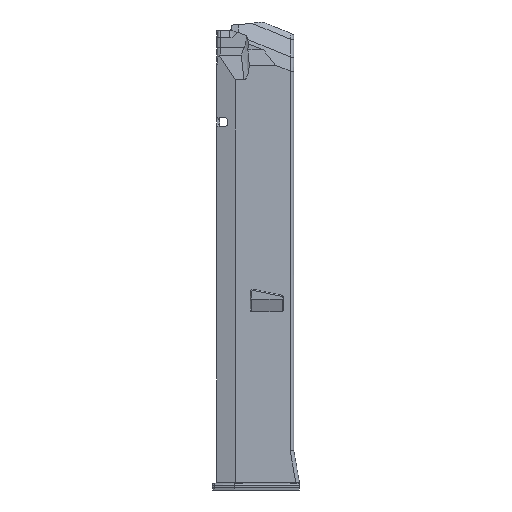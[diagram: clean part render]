
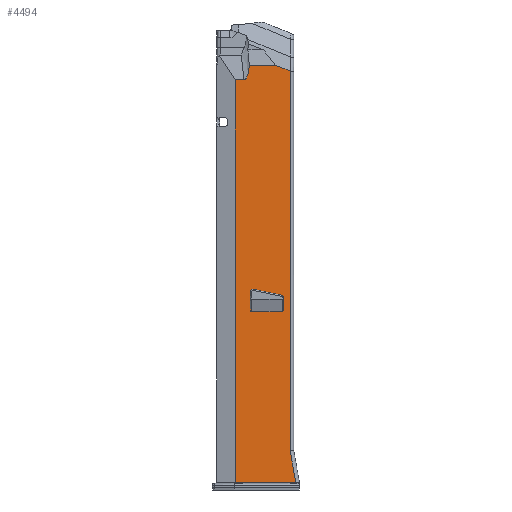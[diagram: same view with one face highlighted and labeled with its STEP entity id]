
A CAD part, left-side view. The second image highlights one B-rep face of the part: STEP entity #4494.
In plain terms, the highlighted planar face has unit normal (-1, 0, 0).
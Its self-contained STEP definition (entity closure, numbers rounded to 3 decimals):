
#103=FACE_BOUND('',#871,.T.);
#232=ELLIPSE('',#4677,1.005,1.);
#234=ELLIPSE('',#4680,1.005,1.);
#236=ELLIPSE('',#4683,1.463,0.503);
#240=ELLIPSE('',#4691,1.463,0.503);
#604=FACE_OUTER_BOUND('',#870,.T.);
#870=EDGE_LOOP('',(#4104,#4105,#4106,#4107,#4108,#4109,#4110,#4111));
#871=EDGE_LOOP('',(#4112,#4113,#4114,#4115,#4116,#4117,#4118,#4119));
#875=LINE('',#5754,#1214);
#882=LINE('',#5841,#1221);
#983=LINE('',#6915,#1322);
#989=LINE('',#6984,#1328);
#994=LINE('',#7002,#1333);
#1074=LINE('',#8695,#1413);
#1077=LINE('',#8703,#1416);
#1082=LINE('',#8725,#1421);
#1085=LINE('',#8741,#1424);
#1175=LINE('',#11174,#1514);
#1211=LINE('',#11465,#1550);
#1214=VECTOR('',#4813,10.);
#1221=VECTOR('',#4826,10.043);
#1322=VECTOR('',#5065,10.05);
#1328=VECTOR('',#5085,10.002);
#1333=VECTOR('',#5098,10.);
#1413=VECTOR('',#5338,10.05);
#1416=VECTOR('',#5343,10.);
#1421=VECTOR('',#5354,10.048);
#1424=VECTOR('',#5363,10.);
#1514=VECTOR('',#5635,10.05);
#1550=VECTOR('',#5731,10.);
#1559=B_SPLINE_CURVE_WITH_KNOTS('',3,(#5826,#5827,#5828,#5829,#5830,#5831,
#5832,#5833,#5834,#5835,#5836,#5837,#5838),.UNSPECIFIED.,.F.,.F.,(4,3,3,
3,4),(0.44,0.612,0.907,1.091,
1.202),.UNSPECIFIED.);
#1712=VERTEX_POINT('',#5748);
#1713=VERTEX_POINT('',#5753);
#1723=VERTEX_POINT('',#5821);
#1724=VERTEX_POINT('',#5840);
#1826=VERTEX_POINT('',#6840);
#1836=VERTEX_POINT('',#6914);
#1842=VERTEX_POINT('',#6982);
#1845=VERTEX_POINT('',#7001);
#1972=VERTEX_POINT('',#8691);
#1973=VERTEX_POINT('',#8693);
#1976=VERTEX_POINT('',#8700);
#1977=VERTEX_POINT('',#8702);
#1979=VERTEX_POINT('',#8717);
#1981=VERTEX_POINT('',#8723);
#1983=VERTEX_POINT('',#8734);
#1985=VERTEX_POINT('',#8739);
#2133=EDGE_CURVE('',#1713,#1712,#875,.T.);
#2146=EDGE_CURVE('',#1723,#1712,#1559,.F.);
#2147=EDGE_CURVE('',#1713,#1724,#882,.T.);
#2311=EDGE_CURVE('',#1826,#1836,#983,.T.);
#2324=EDGE_CURVE('',#1842,#1826,#989,.T.);
#2330=EDGE_CURVE('',#1845,#1836,#994,.T.);
#2510=EDGE_CURVE('',#1973,#1972,#1074,.T.);
#2513=EDGE_CURVE('',#1976,#1977,#1077,.T.);
#2517=EDGE_CURVE('',#1976,#1979,#232,.F.);
#2520=EDGE_CURVE('',#1981,#1979,#1082,.T.);
#2523=EDGE_CURVE('',#1981,#1983,#234,.F.);
#2525=EDGE_CURVE('',#1985,#1983,#1085,.T.);
#2528=EDGE_CURVE('',#1973,#1977,#236,.F.);
#2534=EDGE_CURVE('',#1985,#1972,#240,.F.);
#2744=EDGE_CURVE('',#1845,#1723,#1175,.T.);
#2799=EDGE_CURVE('',#1724,#1842,#1211,.T.);
#4104=ORIENTED_EDGE('',*,*,#2133,.T.);
#4105=ORIENTED_EDGE('',*,*,#2146,.F.);
#4106=ORIENTED_EDGE('',*,*,#2744,.F.);
#4107=ORIENTED_EDGE('',*,*,#2330,.T.);
#4108=ORIENTED_EDGE('',*,*,#2311,.F.);
#4109=ORIENTED_EDGE('',*,*,#2324,.F.);
#4110=ORIENTED_EDGE('',*,*,#2799,.F.);
#4111=ORIENTED_EDGE('',*,*,#2147,.F.);
#4112=ORIENTED_EDGE('',*,*,#2510,.F.);
#4113=ORIENTED_EDGE('',*,*,#2528,.T.);
#4114=ORIENTED_EDGE('',*,*,#2513,.F.);
#4115=ORIENTED_EDGE('',*,*,#2517,.T.);
#4116=ORIENTED_EDGE('',*,*,#2520,.F.);
#4117=ORIENTED_EDGE('',*,*,#2523,.T.);
#4118=ORIENTED_EDGE('',*,*,#2525,.F.);
#4119=ORIENTED_EDGE('',*,*,#2534,.T.);
#4242=PLANE('',#4803);
#4494=ADVANCED_FACE('',(#604,#103),#4242,.T.);
#4677=AXIS2_PLACEMENT_3D('',#8719,#5348,#5349);
#4680=AXIS2_PLACEMENT_3D('',#8736,#5358,#5359);
#4683=AXIS2_PLACEMENT_3D('',#8750,#5367,#5368);
#4691=AXIS2_PLACEMENT_3D('',#8932,#5383,#5384);
#4803=AXIS2_PLACEMENT_3D('',#11466,#5732,#5733);
#4813=DIRECTION('',(0.,1.,0.));
#4826=DIRECTION('',(0.,-0.925,-0.381));
#5065=DIRECTION('',(0.,1.,0.));
#5085=DIRECTION('',(0.,-0.177,-0.984));
#5098=DIRECTION('',(0.,0.,-1.));
#5338=DIRECTION('',(0.,-1.,0.));
#5343=DIRECTION('',(0.,0.,-1.));
#5348=DIRECTION('center_axis',(-1.,0.,0.));
#5349=DIRECTION('ref_axis',(0.,1.,0.));
#5354=DIRECTION('',(0.,0.98,0.198));
#5358=DIRECTION('center_axis',(-1.,0.,0.));
#5359=DIRECTION('ref_axis',(0.,1.,0.));
#5363=DIRECTION('',(0.,0.,1.));
#5367=DIRECTION('center_axis',(-1.,0.,0.));
#5368=DIRECTION('ref_axis',(0.,0.,
-1.));
#5383=DIRECTION('center_axis',(-1.,0.,0.));
#5384=DIRECTION('ref_axis',(0.,0.,-1.));
#5635=DIRECTION('',(0.,-1.,0.));
#5731=DIRECTION('',(0.,0.,-1.));
#5732=DIRECTION('center_axis',(-1.,0.,0.));
#5733=DIRECTION('ref_axis',(0.,0.,1.));
#5748=CARTESIAN_POINT('',(-10.605,2.488,125.254));
#5753=CARTESIAN_POINT('',(-10.605,-8.743,125.254));
#5754=CARTESIAN_POINT('',(-10.605,-7.106,125.254));
#5821=CARTESIAN_POINT('',(-10.605,4.794,118.95));
#5826=CARTESIAN_POINT('Ctrl Pts',(-10.605,2.488,125.254));
#5827=CARTESIAN_POINT('Ctrl Pts',(-10.605,2.551,124.671));
#5828=CARTESIAN_POINT('Ctrl Pts',(-10.605,2.625,124.084));
#5829=CARTESIAN_POINT('Ctrl Pts',(-10.605,2.721,123.473));
#5830=CARTESIAN_POINT('Ctrl Pts',(-10.605,2.885,122.43));
#5831=CARTESIAN_POINT('Ctrl Pts',(-10.605,3.107,121.378));
#5832=CARTESIAN_POINT('Ctrl Pts',(-10.605,3.411,120.551));
#5833=CARTESIAN_POINT('Ctrl Pts',(-10.605,3.6,120.035));
#5834=CARTESIAN_POINT('Ctrl Pts',(-10.605,3.808,119.598));
#5835=CARTESIAN_POINT('Ctrl Pts',(-10.605,4.115,119.28));
#5836=CARTESIAN_POINT('Ctrl Pts',(-10.605,4.301,119.089));
#5837=CARTESIAN_POINT('Ctrl Pts',(-10.605,4.534,118.95));
#5838=CARTESIAN_POINT('Ctrl Pts',(-10.605,4.794,118.95));
#5840=CARTESIAN_POINT('',(-10.605,-14.867,122.73));
#5841=CARTESIAN_POINT('',(-10.605,-32.651,115.4));
#6840=CARTESIAN_POINT('',(-10.605,-17.266,-52.3));
#6914=CARTESIAN_POINT('',(-10.605,8.6,-52.3));
#6915=CARTESIAN_POINT('',(-10.605,-8.214,-52.3));
#6982=CARTESIAN_POINT('',(-10.605,-14.867,-38.933));
#6984=CARTESIAN_POINT('',(-10.605,-16.431,-47.651));
#7001=CARTESIAN_POINT('',(-10.605,8.6,118.95));
#7002=CARTESIAN_POINT('',(-10.605,8.6,6.3));
#8691=CARTESIAN_POINT('',(-10.605,-11.532,20.2));
#8693=CARTESIAN_POINT('',(-10.605,1.533,20.2));
#8695=CARTESIAN_POINT('',(-10.605,-14.205,20.2));
#8700=CARTESIAN_POINT('',(-10.605,2.035,28.824));
#8702=CARTESIAN_POINT('',(-10.605,2.035,21.663));
#8703=CARTESIAN_POINT('',(-10.605,2.035,13.25));
#8717=CARTESIAN_POINT('',(-10.605,0.83,29.804));
#8719=CARTESIAN_POINT('Origin',(-10.605,1.03,28.824));
#8723=CARTESIAN_POINT('',(-10.605,-11.23,27.363));
#8725=CARTESIAN_POINT('',(-10.605,-9.135,27.787));
#8734=CARTESIAN_POINT('',(-10.605,-12.035,26.383));
#8736=CARTESIAN_POINT('Origin',(-10.605,-11.03,26.383));
#8739=CARTESIAN_POINT('',(-10.605,-12.035,21.663));
#8741=CARTESIAN_POINT('',(-10.605,-12.035,16.75));
#8750=CARTESIAN_POINT('Origin',(-10.605,1.533,21.663));
#8932=CARTESIAN_POINT('Origin',(-10.605,-11.532,21.663));
#11174=CARTESIAN_POINT('',(-10.605,-0.043,118.95));
#11465=CARTESIAN_POINT('',(-10.605,-14.867,-49.3));
#11466=CARTESIAN_POINT('Origin',(-10.605,-16.374,6.3));
